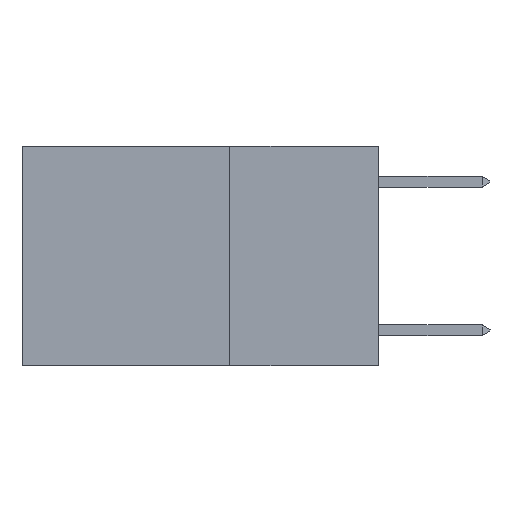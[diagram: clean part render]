
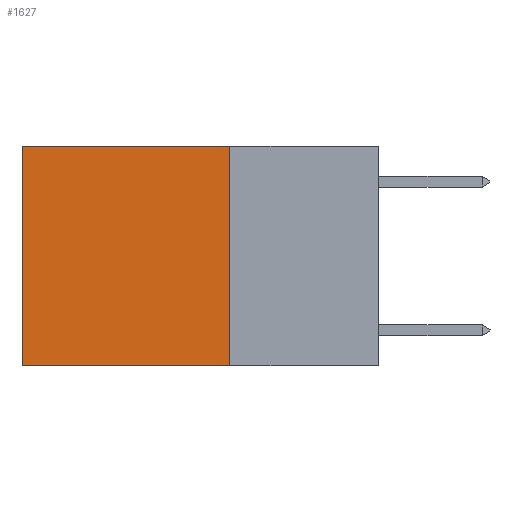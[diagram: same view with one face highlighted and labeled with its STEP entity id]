
A CAD part, left-side view. The second image highlights one B-rep face of the part: STEP entity #1627.
In plain terms, the highlighted planar face has unit normal (-1, 0, 0).
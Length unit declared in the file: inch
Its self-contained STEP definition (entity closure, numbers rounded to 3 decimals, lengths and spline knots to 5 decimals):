
#51 = VERTEX_POINT ( 'NONE', #6348 ) ;
#673 = CARTESIAN_POINT ( 'NONE',  ( 0.2625, 0.25, 0. ) ) ;
#729 = DIRECTION ( 'NONE',  ( 0., 1., 0. ) ) ;
#781 = DIRECTION ( 'NONE',  ( 0., 0., -1. ) ) ;
#1080 = DIRECTION ( 'NONE',  ( 0., 0., -1. ) ) ;
#1627 = ADVANCED_FACE ( 'NONE', ( #8140 ), #8562, .F. ) ;
#2001 = ORIENTED_EDGE ( 'NONE', *, *, #3538, .T. ) ;
#2250 = EDGE_LOOP ( 'NONE', ( #9366, #5008, #7043, #2001 ) ) ;
#2396 = CARTESIAN_POINT ( 'NONE',  ( 0.2625, 0.6, -0.37 ) ) ;
#3109 = VECTOR ( 'NONE', #729, 39.37008 ) ;
#3476 = VERTEX_POINT ( 'NONE', #11194 ) ;
#3538 = EDGE_CURVE ( 'NONE', #51, #3476, #5467, .T. ) ;
#3649 = VERTEX_POINT ( 'NONE', #10083 ) ;
#4208 = EDGE_CURVE ( 'NONE', #3649, #8833, #5170, .T. ) ;
#5008 = ORIENTED_EDGE ( 'NONE', *, *, #4208, .F. ) ;
#5120 = EDGE_CURVE ( 'NONE', #3476, #8833, #6542, .T. ) ;
#5170 = LINE ( 'NONE', #9233, #5848 ) ;
#5274 = LINE ( 'NONE', #11469, #8949 ) ;
#5467 = LINE ( 'NONE', #673, #3109 ) ;
#5848 = VECTOR ( 'NONE', #10138, 39.37008 ) ;
#6161 = DIRECTION ( 'NONE',  ( 1., 0., 0. ) ) ;
#6348 = CARTESIAN_POINT ( 'NONE',  ( 0.2625, 0.25, 0. ) ) ;
#6542 = LINE ( 'NONE', #7732, #8088 ) ;
#7043 = ORIENTED_EDGE ( 'NONE', *, *, #9973, .F. ) ;
#7732 = CARTESIAN_POINT ( 'NONE',  ( 0.2625, 0.6, 0. ) ) ;
#8088 = VECTOR ( 'NONE', #11242, 39.37008 ) ;
#8140 = FACE_OUTER_BOUND ( 'NONE', #2250, .T. ) ;
#8562 = PLANE ( 'NONE',  #10099 ) ;
#8833 = VERTEX_POINT ( 'NONE', #2396 ) ;
#8949 = VECTOR ( 'NONE', #781, 39.37008 ) ;
#9233 = CARTESIAN_POINT ( 'NONE',  ( 0.2625, 0.25, -0.37 ) ) ;
#9366 = ORIENTED_EDGE ( 'NONE', *, *, #5120, .T. ) ;
#9973 = EDGE_CURVE ( 'NONE', #51, #3649, #5274, .T. ) ;
#10083 = CARTESIAN_POINT ( 'NONE',  ( 0.2625, 0.25, -0.37 ) ) ;
#10099 = AXIS2_PLACEMENT_3D ( 'NONE', #10558, #6161, #1080 ) ;
#10138 = DIRECTION ( 'NONE',  ( 0., 1., 0. ) ) ;
#10558 = CARTESIAN_POINT ( 'NONE',  ( 0.2625, 0.25, 0. ) ) ;
#11194 = CARTESIAN_POINT ( 'NONE',  ( 0.2625, 0.6, 0. ) ) ;
#11242 = DIRECTION ( 'NONE',  ( 0., 0., -1. ) ) ;
#11469 = CARTESIAN_POINT ( 'NONE',  ( 0.2625, 0.25, 0. ) ) ;
